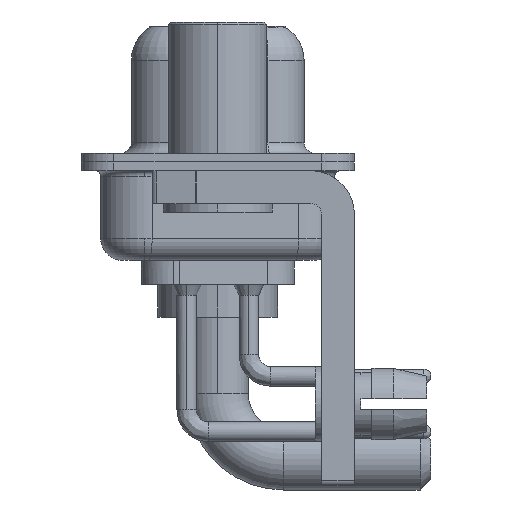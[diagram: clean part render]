
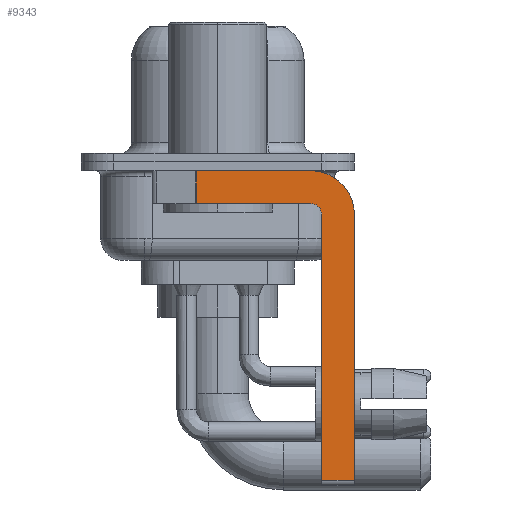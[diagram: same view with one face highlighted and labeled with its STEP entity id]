
A CAD part, left-side view. The second image highlights one B-rep face of the part: STEP entity #9343.
In plain terms, the highlighted planar face has unit normal (-1, 0, 0).
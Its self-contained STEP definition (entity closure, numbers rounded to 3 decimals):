
#49 = EDGE_LOOP ( 'NONE', ( #12120, #15153, #21047, #19153, #14665, #10696, #656, #11746 ) ) ;
#152 = CARTESIAN_POINT ( 'NONE',  ( -2.9, 0.978, -1.9 ) ) ;
#525 = EDGE_CURVE ( 'NONE', #9818, #11594, #6869, .T. ) ;
#637 = AXIS2_PLACEMENT_3D ( 'NONE', #18844, #18410, #11736 ) ;
#656 = ORIENTED_EDGE ( 'NONE', *, *, #7163, .F. ) ;
#1358 = CARTESIAN_POINT ( 'NONE',  ( -2.9, -6.25, -2.4 ) ) ;
#1569 = CARTESIAN_POINT ( 'NONE',  ( -2.9, -4.25, -14.55 ) ) ;
#2305 = LINE ( 'NONE', #14391, #3898 ) ;
#2925 = AXIS2_PLACEMENT_3D ( 'NONE', #16231, #5582, #15897 ) ;
#3213 = VECTOR ( 'NONE', #16475, 1000. ) ;
#3220 = DIRECTION ( 'NONE',  ( 0., 0., 1. ) ) ;
#3336 = CARTESIAN_POINT ( 'NONE',  ( -2.9, -4.75, -14.8 ) ) ;
#3738 = CARTESIAN_POINT ( 'NONE',  ( -2.9, -4.25, -1.9 ) ) ;
#3898 = VECTOR ( 'NONE', #12518, 1000. ) ;
#3971 = LINE ( 'NONE', #4183, #9588 ) ;
#4183 = CARTESIAN_POINT ( 'NONE',  ( -2.9, -6.25, -2.4 ) ) ;
#4552 = VERTEX_POINT ( 'NONE', #12731 ) ;
#5513 = VECTOR ( 'NONE', #6459, 1000. ) ;
#5569 = EDGE_CURVE ( 'NONE', #4552, #12773, #8514, .T. ) ;
#5582 = DIRECTION ( 'NONE',  ( 1., 0., 0. ) ) ;
#6459 = DIRECTION ( 'NONE',  ( 0., -1., 0. ) ) ;
#6869 = LINE ( 'NONE', #3738, #11988 ) ;
#6890 = EDGE_CURVE ( 'NONE', #8396, #18806, #18445, .T. ) ;
#7130 = EDGE_CURVE ( 'NONE', #10852, #4552, #2305, .T. ) ;
#7163 = EDGE_CURVE ( 'NONE', #12773, #9793, #3971, .T. ) ;
#7493 = DIRECTION ( 'NONE',  ( -1., 0., 0. ) ) ;
#7584 = LINE ( 'NONE', #14353, #3213 ) ;
#7686 = FACE_OUTER_BOUND ( 'NONE', #49, .T. ) ;
#8036 = AXIS2_PLACEMENT_3D ( 'NONE', #19069, #7493, #19382 ) ;
#8396 = VERTEX_POINT ( 'NONE', #9204 ) ;
#8514 = CIRCLE ( 'NONE', #637, 2. ) ;
#9204 = CARTESIAN_POINT ( 'NONE',  ( -2.9, -4.75, -14.55 ) ) ;
#9343 = ADVANCED_FACE ( 'NONE', ( #7686 ), #9371, .F. ) ;
#9371 = PLANE ( 'NONE',  #2925 ) ;
#9588 = VECTOR ( 'NONE', #14292, 1000. ) ;
#9793 = VERTEX_POINT ( 'NONE', #20243 ) ;
#9818 = VERTEX_POINT ( 'NONE', #16905 ) ;
#10512 = DIRECTION ( 'NONE',  ( 0., 1., 0. ) ) ;
#10696 = ORIENTED_EDGE ( 'NONE', *, *, #14417, .T. ) ;
#10852 = VERTEX_POINT ( 'NONE', #12747 ) ;
#11594 = VERTEX_POINT ( 'NONE', #152 ) ;
#11736 = DIRECTION ( 'NONE',  ( 0., 0., -1. ) ) ;
#11746 = ORIENTED_EDGE ( 'NONE', *, *, #5569, .F. ) ;
#11988 = VECTOR ( 'NONE', #10512, 1000. ) ;
#12120 = ORIENTED_EDGE ( 'NONE', *, *, #7130, .F. ) ;
#12518 = DIRECTION ( 'NONE',  ( 0., -1., 0. ) ) ;
#12731 = CARTESIAN_POINT ( 'NONE',  ( -2.9, -4.25, -0.4 ) ) ;
#12747 = CARTESIAN_POINT ( 'NONE',  ( -2.9, 0.978, -0.4 ) ) ;
#12773 = VERTEX_POINT ( 'NONE', #1358 ) ;
#13363 = CIRCLE ( 'NONE', #8036, 0.5 ) ;
#13890 = EDGE_CURVE ( 'NONE', #18806, #9818, #13363, .T. ) ;
#14292 = DIRECTION ( 'NONE',  ( 0., 0., -1. ) ) ;
#14353 = CARTESIAN_POINT ( 'NONE',  ( -2.9, 0.978, -1.9 ) ) ;
#14391 = CARTESIAN_POINT ( 'NONE',  ( -2.9, 3., -0.4 ) ) ;
#14417 = EDGE_CURVE ( 'NONE', #8396, #9793, #20219, .T. ) ;
#14665 = ORIENTED_EDGE ( 'NONE', *, *, #6890, .F. ) ;
#15153 = ORIENTED_EDGE ( 'NONE', *, *, #19965, .T. ) ;
#15897 = DIRECTION ( 'NONE',  ( 0., 0., -1. ) ) ;
#16231 = CARTESIAN_POINT ( 'NONE',  ( -2.9, -4.25, -2.4 ) ) ;
#16475 = DIRECTION ( 'NONE',  ( 0., 0., -1. ) ) ;
#16905 = CARTESIAN_POINT ( 'NONE',  ( -2.9, -4.25, -1.9 ) ) ;
#17017 = VECTOR ( 'NONE', #3220, 1000. ) ;
#18410 = DIRECTION ( 'NONE',  ( 1., 0., 0. ) ) ;
#18445 = LINE ( 'NONE', #3336, #17017 ) ;
#18806 = VERTEX_POINT ( 'NONE', #20641 ) ;
#18844 = CARTESIAN_POINT ( 'NONE',  ( -2.9, -4.25, -2.4 ) ) ;
#19069 = CARTESIAN_POINT ( 'NONE',  ( -2.9, -4.25, -2.4 ) ) ;
#19153 = ORIENTED_EDGE ( 'NONE', *, *, #13890, .F. ) ;
#19382 = DIRECTION ( 'NONE',  ( 0., 0., 1. ) ) ;
#19965 = EDGE_CURVE ( 'NONE', #10852, #11594, #7584, .T. ) ;
#20219 = LINE ( 'NONE', #1569, #5513 ) ;
#20243 = CARTESIAN_POINT ( 'NONE',  ( -2.9, -6.25, -14.55 ) ) ;
#20641 = CARTESIAN_POINT ( 'NONE',  ( -2.9, -4.75, -2.4 ) ) ;
#21047 = ORIENTED_EDGE ( 'NONE', *, *, #525, .F. ) ;
